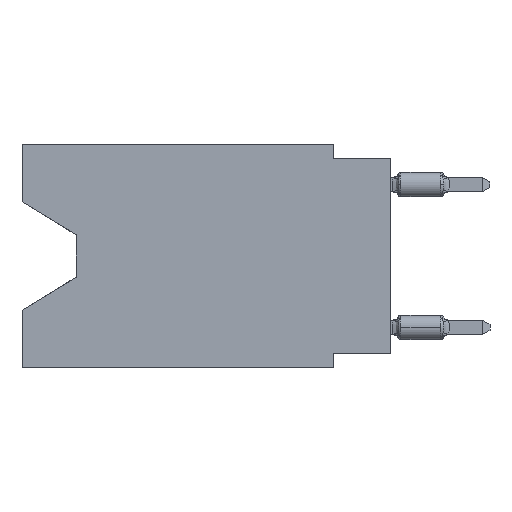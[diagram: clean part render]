
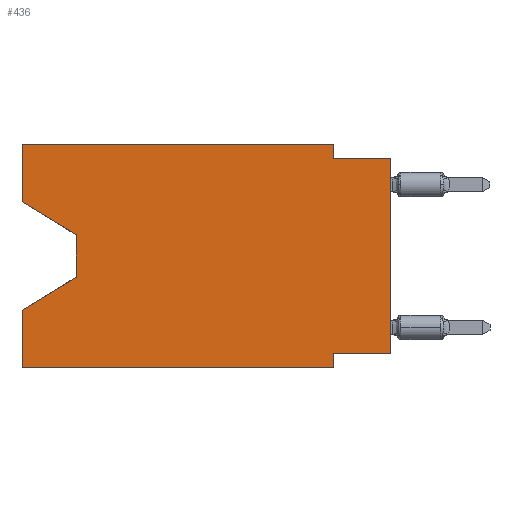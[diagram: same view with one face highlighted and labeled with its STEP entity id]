
A CAD part, left-side view. The second image highlights one B-rep face of the part: STEP entity #436.
In plain terms, the highlighted planar face has unit normal (-1, 0, 0).
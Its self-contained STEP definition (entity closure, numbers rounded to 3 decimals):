
#3 = VERTEX_POINT ( 'NONE', #1795 ) ;
#71 = DIRECTION ( 'NONE',  ( 0., 0., -1. ) ) ;
#92 = CARTESIAN_POINT ( 'NONE',  ( 0., 0., -9.271 ) ) ;
#172 = ORIENTED_EDGE ( 'NONE', *, *, #14988, .T. ) ;
#305 = VERTEX_POINT ( 'NONE', #5614 ) ;
#436 = ADVANCED_FACE ( 'NONE', ( #18659 ), #15219, .F. ) ;
#663 = CARTESIAN_POINT ( 'NONE',  ( 0., 13.97, -4.013 ) ) ;
#958 = VECTOR ( 'NONE', #2478, 1000. ) ;
#1160 = CARTESIAN_POINT ( 'NONE',  ( 0., 2.54, 0. ) ) ;
#1208 = LINE ( 'NONE', #19910, #16403 ) ;
#1234 = DIRECTION ( 'NONE',  ( 0., 0., -1. ) ) ;
#1261 = CARTESIAN_POINT ( 'NONE',  ( 0., 16.383, -9.906 ) ) ;
#1795 = CARTESIAN_POINT ( 'NONE',  ( 0., 16.383, -7.36 ) ) ;
#1913 = VECTOR ( 'NONE', #14675, 1000. ) ;
#2008 = VECTOR ( 'NONE', #19667, 1000. ) ;
#2478 = DIRECTION ( 'NONE',  ( 0., 0., 1. ) ) ;
#2574 = DIRECTION ( 'NONE',  ( 0., 0., -1. ) ) ;
#2612 = VERTEX_POINT ( 'NONE', #15421 ) ;
#2732 = EDGE_CURVE ( 'NONE', #13119, #2612, #4051, .T. ) ;
#2757 = LINE ( 'NONE', #1261, #3828 ) ;
#2954 = VERTEX_POINT ( 'NONE', #11938 ) ;
#3024 = ORIENTED_EDGE ( 'NONE', *, *, #3365, .F. ) ;
#3107 = LINE ( 'NONE', #92, #3493 ) ;
#3319 = CARTESIAN_POINT ( 'NONE',  ( 0., 16.383, -2.546 ) ) ;
#3365 = EDGE_CURVE ( 'NONE', #19776, #5953, #1208, .T. ) ;
#3384 = LINE ( 'NONE', #15705, #13657 ) ;
#3452 = VERTEX_POINT ( 'NONE', #14036 ) ;
#3493 = VECTOR ( 'NONE', #10876, 1000. ) ;
#3661 = CARTESIAN_POINT ( 'NONE',  ( 0., 2.54, -9.906 ) ) ;
#3828 = VECTOR ( 'NONE', #8904, 1000. ) ;
#4051 = LINE ( 'NONE', #13357, #1913 ) ;
#4075 = CARTESIAN_POINT ( 'NONE',  ( 0., 0., -0.635 ) ) ;
#4129 = ORIENTED_EDGE ( 'NONE', *, *, #2732, .F. ) ;
#4167 = CARTESIAN_POINT ( 'NONE',  ( 0., 16.383, -2.546 ) ) ;
#4283 = EDGE_CURVE ( 'NONE', #13620, #3452, #18228, .T. ) ;
#4573 = ORIENTED_EDGE ( 'NONE', *, *, #4283, .F. ) ;
#4752 = EDGE_CURVE ( 'NONE', #305, #3, #19452, .T. ) ;
#4799 = DIRECTION ( 'NONE',  ( 1., 0., 0. ) ) ;
#5316 = LINE ( 'NONE', #11468, #958 ) ;
#5422 = VECTOR ( 'NONE', #16394, 1000. ) ;
#5529 = EDGE_CURVE ( 'NONE', #3452, #12534, #14810, .T. ) ;
#5589 = CARTESIAN_POINT ( 'NONE',  ( 0., 13.97, -5.893 ) ) ;
#5614 = CARTESIAN_POINT ( 'NONE',  ( 0., 13.97, -5.893 ) ) ;
#5953 = VERTEX_POINT ( 'NONE', #3661 ) ;
#6046 = DIRECTION ( 'NONE',  ( 0., 0., -1. ) ) ;
#6077 = LINE ( 'NONE', #16887, #10973 ) ;
#6103 = VECTOR ( 'NONE', #9460, 1000. ) ;
#6381 = ORIENTED_EDGE ( 'NONE', *, *, #13336, .T. ) ;
#6807 = ORIENTED_EDGE ( 'NONE', *, *, #9264, .T. ) ;
#7115 = EDGE_CURVE ( 'NONE', #2612, #13620, #3384, .T. ) ;
#8400 = CARTESIAN_POINT ( 'NONE',  ( 0., 2.54, 0. ) ) ;
#8503 = EDGE_CURVE ( 'NONE', #2954, #3, #8592, .T. ) ;
#8572 = ORIENTED_EDGE ( 'NONE', *, *, #19270, .T. ) ;
#8592 = LINE ( 'NONE', #13570, #9933 ) ;
#8896 = DIRECTION ( 'NONE',  ( 0., 0., 1. ) ) ;
#8904 = DIRECTION ( 'NONE',  ( 0., -1., 0. ) ) ;
#9264 = EDGE_CURVE ( 'NONE', #17269, #12534, #5316, .T. ) ;
#9460 = DIRECTION ( 'NONE',  ( 0., -0.855, -0.519 ) ) ;
#9933 = VECTOR ( 'NONE', #8896, 1000. ) ;
#9977 = EDGE_LOOP ( 'NONE', ( #8572, #172, #13877, #17357, #6381, #3024, #11329, #6807, #14162, #4573, #17153, #4129 ) ) ;
#10556 = VECTOR ( 'NONE', #2574, 1000. ) ;
#10876 = DIRECTION ( 'NONE',  ( 0., 1., 0. ) ) ;
#10973 = VECTOR ( 'NONE', #1234, 1000. ) ;
#11329 = ORIENTED_EDGE ( 'NONE', *, *, #18015, .F. ) ;
#11468 = CARTESIAN_POINT ( 'NONE',  ( 0., 0., 0. ) ) ;
#11938 = CARTESIAN_POINT ( 'NONE',  ( 0., 16.383, -9.906 ) ) ;
#11952 = CARTESIAN_POINT ( 'NONE',  ( 0., 2.54, -9.271 ) ) ;
#12497 = LINE ( 'NONE', #3319, #6103 ) ;
#12534 = VERTEX_POINT ( 'NONE', #18481 ) ;
#12770 = CARTESIAN_POINT ( 'NONE',  ( 0., 0., -9.271 ) ) ;
#13119 = VERTEX_POINT ( 'NONE', #4167 ) ;
#13336 = EDGE_CURVE ( 'NONE', #2954, #5953, #2757, .T. ) ;
#13357 = CARTESIAN_POINT ( 'NONE',  ( 0., 16.383, 0. ) ) ;
#13570 = CARTESIAN_POINT ( 'NONE',  ( 0., 16.383, 0. ) ) ;
#13620 = VERTEX_POINT ( 'NONE', #8400 ) ;
#13657 = VECTOR ( 'NONE', #13683, 1000. ) ;
#13683 = DIRECTION ( 'NONE',  ( 0., -1., 0. ) ) ;
#13877 = ORIENTED_EDGE ( 'NONE', *, *, #4752, .T. ) ;
#14036 = CARTESIAN_POINT ( 'NONE',  ( 0., 2.54, -0.635 ) ) ;
#14162 = ORIENTED_EDGE ( 'NONE', *, *, #5529, .F. ) ;
#14675 = DIRECTION ( 'NONE',  ( 0., 0., 1. ) ) ;
#14810 = LINE ( 'NONE', #4075, #2008 ) ;
#14925 = VERTEX_POINT ( 'NONE', #663 ) ;
#14988 = EDGE_CURVE ( 'NONE', #14925, #305, #6077, .T. ) ;
#15219 = PLANE ( 'NONE',  #16347 ) ;
#15421 = CARTESIAN_POINT ( 'NONE',  ( 0., 16.383, 0. ) ) ;
#15705 = CARTESIAN_POINT ( 'NONE',  ( 0., 16.383, 0. ) ) ;
#16347 = AXIS2_PLACEMENT_3D ( 'NONE', #19870, #4799, #71 ) ;
#16394 = DIRECTION ( 'NONE',  ( 0., 0.855, -0.519 ) ) ;
#16403 = VECTOR ( 'NONE', #6046, 1000. ) ;
#16887 = CARTESIAN_POINT ( 'NONE',  ( 0., 13.97, -4.013 ) ) ;
#17153 = ORIENTED_EDGE ( 'NONE', *, *, #7115, .F. ) ;
#17269 = VERTEX_POINT ( 'NONE', #12770 ) ;
#17357 = ORIENTED_EDGE ( 'NONE', *, *, #8503, .F. ) ;
#18015 = EDGE_CURVE ( 'NONE', #17269, #19776, #3107, .T. ) ;
#18228 = LINE ( 'NONE', #1160, #10556 ) ;
#18481 = CARTESIAN_POINT ( 'NONE',  ( 0., 0., -0.635 ) ) ;
#18659 = FACE_OUTER_BOUND ( 'NONE', #9977, .T. ) ;
#19270 = EDGE_CURVE ( 'NONE', #13119, #14925, #12497, .T. ) ;
#19452 = LINE ( 'NONE', #5589, #5422 ) ;
#19667 = DIRECTION ( 'NONE',  ( 0., -1., 0. ) ) ;
#19776 = VERTEX_POINT ( 'NONE', #11952 ) ;
#19870 = CARTESIAN_POINT ( 'NONE',  ( 0., 16.383, 0. ) ) ;
#19910 = CARTESIAN_POINT ( 'NONE',  ( 0., 2.54, -9.906 ) ) ;
